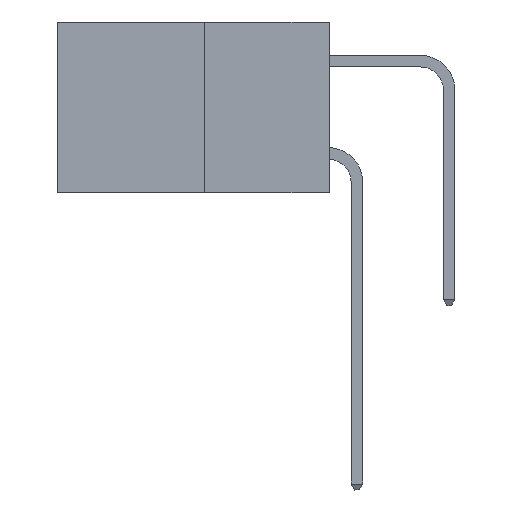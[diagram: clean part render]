
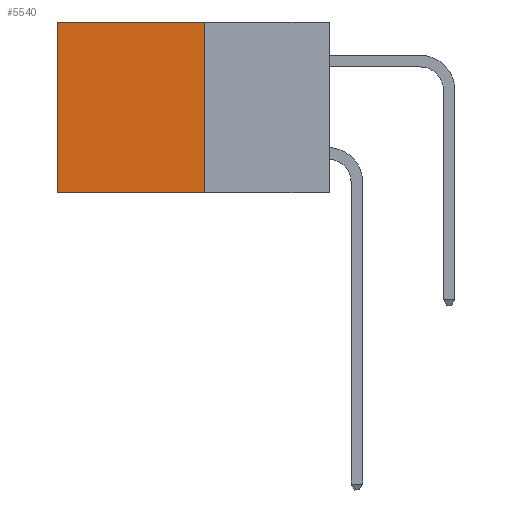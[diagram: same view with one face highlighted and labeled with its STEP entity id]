
A CAD part, left-side view. The second image highlights one B-rep face of the part: STEP entity #5540.
In plain terms, the highlighted planar face has unit normal (-1, 0, 0).
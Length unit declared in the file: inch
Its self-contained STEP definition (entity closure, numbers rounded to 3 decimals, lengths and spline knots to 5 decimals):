
#569 = CARTESIAN_POINT ( 'NONE',  ( 0.277, 0.27, -0.37 ) ) ;
#829 = DIRECTION ( 'NONE',  ( 0., 1., 0. ) ) ;
#1289 = EDGE_CURVE ( 'NONE', #29985, #12255, #16072, .T. ) ;
#4726 = LINE ( 'NONE', #10632, #30525 ) ;
#5540 = ADVANCED_FACE ( 'NONE', ( #17931 ), #19430, .F. ) ;
#5686 = DIRECTION ( 'NONE',  ( 0., 1., 0. ) ) ;
#7519 = EDGE_CURVE ( 'NONE', #12255, #28413, #11182, .T. ) ;
#7962 = ORIENTED_EDGE ( 'NONE', *, *, #7519, .F. ) ;
#8117 = EDGE_CURVE ( 'NONE', #10590, #28413, #18184, .T. ) ;
#8587 = CARTESIAN_POINT ( 'NONE',  ( 0.277, 0.27, -0.37 ) ) ;
#10398 = VECTOR ( 'NONE', #829, 39.37008 ) ;
#10590 = VERTEX_POINT ( 'NONE', #27501 ) ;
#10632 = CARTESIAN_POINT ( 'NONE',  ( 0.277, 0.27, 0. ) ) ;
#11182 = LINE ( 'NONE', #569, #10398 ) ;
#12255 = VERTEX_POINT ( 'NONE', #8587 ) ;
#12312 = VECTOR ( 'NONE', #25752, 39.37008 ) ;
#15821 = CARTESIAN_POINT ( 'NONE',  ( 0.277, 0.59, -0.37 ) ) ;
#15845 = EDGE_CURVE ( 'NONE', #29985, #10590, #4726, .T. ) ;
#16072 = LINE ( 'NONE', #20647, #28590 ) ;
#17931 = FACE_OUTER_BOUND ( 'NONE', #27400, .T. ) ;
#18184 = LINE ( 'NONE', #15821, #12312 ) ;
#18414 = DIRECTION ( 'NONE',  ( 0., 0., -1. ) ) ;
#18661 = ORIENTED_EDGE ( 'NONE', *, *, #1289, .F. ) ;
#19354 = DIRECTION ( 'NONE',  ( 0., 0., -1. ) ) ;
#19358 = DIRECTION ( 'NONE',  ( 1., 0., 0. ) ) ;
#19430 = PLANE ( 'NONE',  #26716 ) ;
#19892 = CARTESIAN_POINT ( 'NONE',  ( 0.277, 0.27, -0.37 ) ) ;
#20411 = ORIENTED_EDGE ( 'NONE', *, *, #8117, .T. ) ;
#20647 = CARTESIAN_POINT ( 'NONE',  ( 0.277, 0.27, -0.37 ) ) ;
#23760 = ORIENTED_EDGE ( 'NONE', *, *, #15845, .T. ) ;
#25752 = DIRECTION ( 'NONE',  ( 0., 0., -1. ) ) ;
#26716 = AXIS2_PLACEMENT_3D ( 'NONE', #19892, #19358, #19354 ) ;
#27400 = EDGE_LOOP ( 'NONE', ( #20411, #7962, #18661, #23760 ) ) ;
#27501 = CARTESIAN_POINT ( 'NONE',  ( 0.277, 0.59, 0. ) ) ;
#28413 = VERTEX_POINT ( 'NONE', #28966 ) ;
#28590 = VECTOR ( 'NONE', #18414, 39.37008 ) ;
#28966 = CARTESIAN_POINT ( 'NONE',  ( 0.277, 0.59, -0.37 ) ) ;
#29957 = CARTESIAN_POINT ( 'NONE',  ( 0.277, 0.27, 0. ) ) ;
#29985 = VERTEX_POINT ( 'NONE', #29957 ) ;
#30525 = VECTOR ( 'NONE', #5686, 39.37008 ) ;
